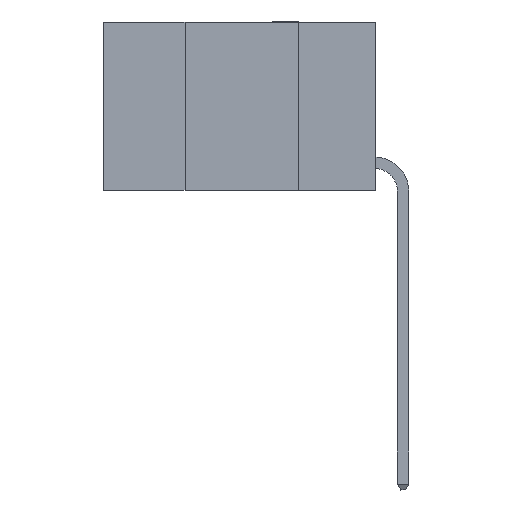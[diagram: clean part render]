
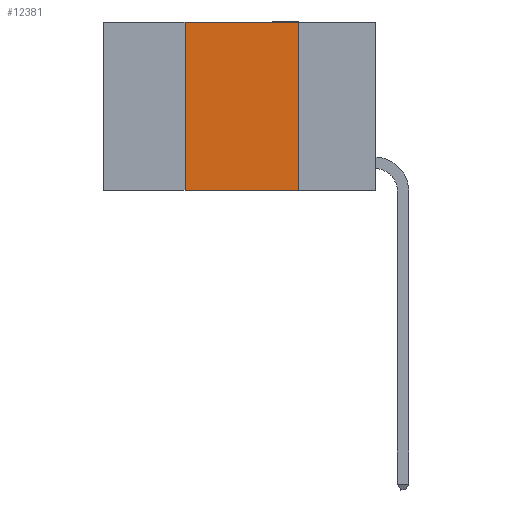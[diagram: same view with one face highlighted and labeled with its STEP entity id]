
A CAD part, left-side view. The second image highlights one B-rep face of the part: STEP entity #12381.
In plain terms, the highlighted planar face has unit normal (-1, 0, 0).
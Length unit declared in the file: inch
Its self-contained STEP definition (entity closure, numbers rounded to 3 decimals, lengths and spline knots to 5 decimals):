
#572 = FACE_OUTER_BOUND ( 'NONE', #12173, .T. ) ;
#724 = VERTEX_POINT ( 'NONE', #3614 ) ;
#792 = VECTOR ( 'NONE', #2665, 39.37008 ) ;
#893 = EDGE_CURVE ( 'NONE', #10988, #12380, #12699, .T. ) ;
#999 = ORIENTED_EDGE ( 'NONE', *, *, #893, .F. ) ;
#1014 = CARTESIAN_POINT ( 'NONE',  ( 0., 0.17, -0.37 ) ) ;
#1094 = CARTESIAN_POINT ( 'NONE',  ( 0., 0.42, -0.37 ) ) ;
#1340 = DIRECTION ( 'NONE',  ( 0., 0., -1. ) ) ;
#1757 = PLANE ( 'NONE',  #3412 ) ;
#2620 = CARTESIAN_POINT ( 'NONE',  ( 0., 0.42, 0. ) ) ;
#2665 = DIRECTION ( 'NONE',  ( 0., -1., 0. ) ) ;
#2967 = VECTOR ( 'NONE', #1340, 39.37008 ) ;
#3309 = VECTOR ( 'NONE', #9786, 39.37008 ) ;
#3412 = AXIS2_PLACEMENT_3D ( 'NONE', #9788, #6765, #6647 ) ;
#3614 = CARTESIAN_POINT ( 'NONE',  ( 0., 0.17, 0. ) ) ;
#3951 = VERTEX_POINT ( 'NONE', #1014 ) ;
#4126 = CARTESIAN_POINT ( 'NONE',  ( 0., 0.17, 0. ) ) ;
#5110 = LINE ( 'NONE', #4126, #2967 ) ;
#5128 = ORIENTED_EDGE ( 'NONE', *, *, #12943, .T. ) ;
#5264 = DIRECTION ( 'NONE',  ( 0., -1., 0. ) ) ;
#5770 = CARTESIAN_POINT ( 'NONE',  ( 0., 0.42, 0. ) ) ;
#6647 = DIRECTION ( 'NONE',  ( 0., 0., -1. ) ) ;
#6765 = DIRECTION ( 'NONE',  ( 1., 0., 0. ) ) ;
#7246 = LINE ( 'NONE', #8534, #7814 ) ;
#7644 = ORIENTED_EDGE ( 'NONE', *, *, #7816, .F. ) ;
#7814 = VECTOR ( 'NONE', #5264, 39.37008 ) ;
#7816 = EDGE_CURVE ( 'NONE', #12380, #724, #7246, .T. ) ;
#7969 = ORIENTED_EDGE ( 'NONE', *, *, #8111, .F. ) ;
#8111 = EDGE_CURVE ( 'NONE', #724, #3951, #5110, .T. ) ;
#8534 = CARTESIAN_POINT ( 'NONE',  ( 0., 0.6, 0. ) ) ;
#9432 = LINE ( 'NONE', #11455, #792 ) ;
#9786 = DIRECTION ( 'NONE',  ( 0., 0., 1. ) ) ;
#9788 = CARTESIAN_POINT ( 'NONE',  ( 0., 0.6, 0. ) ) ;
#10988 = VERTEX_POINT ( 'NONE', #1094 ) ;
#11455 = CARTESIAN_POINT ( 'NONE',  ( 0., 0.6, -0.37 ) ) ;
#12173 = EDGE_LOOP ( 'NONE', ( #7969, #7644, #999, #5128 ) ) ;
#12380 = VERTEX_POINT ( 'NONE', #2620 ) ;
#12381 = ADVANCED_FACE ( 'NONE', ( #572 ), #1757, .F. ) ;
#12699 = LINE ( 'NONE', #5770, #3309 ) ;
#12943 = EDGE_CURVE ( 'NONE', #10988, #3951, #9432, .T. ) ;
